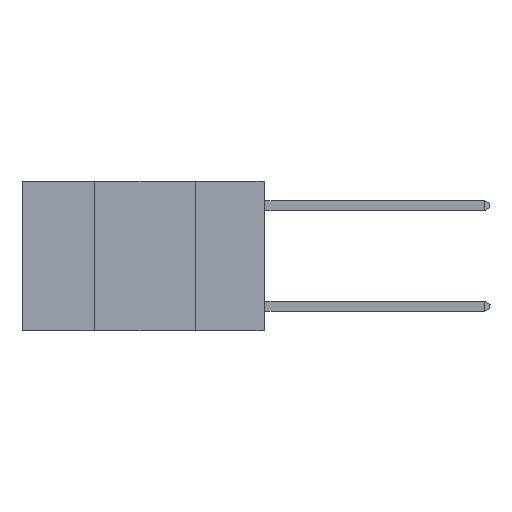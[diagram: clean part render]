
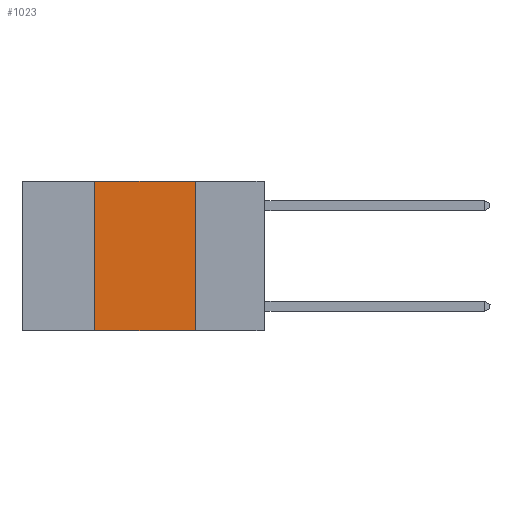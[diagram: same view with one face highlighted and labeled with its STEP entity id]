
A CAD part, left-side view. The second image highlights one B-rep face of the part: STEP entity #1023.
In plain terms, the highlighted planar face has unit normal (-1, 0, 0).
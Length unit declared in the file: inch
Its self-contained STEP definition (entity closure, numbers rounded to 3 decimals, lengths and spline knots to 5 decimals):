
#689 = VERTEX_POINT ( 'NONE', #1444 ) ;
#740 = PLANE ( 'NONE',  #11477 ) ;
#893 = ORIENTED_EDGE ( 'NONE', *, *, #12633, .T. ) ;
#1023 = ADVANCED_FACE ( 'NONE', ( #6993 ), #740, .F. ) ;
#1025 = LINE ( 'NONE', #11976, #3713 ) ;
#1444 = CARTESIAN_POINT ( 'NONE',  ( 0., 0.17, -0.37 ) ) ;
#2032 = VERTEX_POINT ( 'NONE', #9055 ) ;
#2495 = VERTEX_POINT ( 'NONE', #12577 ) ;
#2606 = DIRECTION ( 'NONE',  ( 0., 0., -1. ) ) ;
#3270 = DIRECTION ( 'NONE',  ( 0., -1., 0. ) ) ;
#3518 = DIRECTION ( 'NONE',  ( 1., 0., 0. ) ) ;
#3713 = VECTOR ( 'NONE', #3270, 39.37008 ) ;
#4757 = VECTOR ( 'NONE', #5237, 39.37008 ) ;
#5237 = DIRECTION ( 'NONE',  ( 0., 0., 1. ) ) ;
#6869 = DIRECTION ( 'NONE',  ( 0., 0., -1. ) ) ;
#6993 = FACE_OUTER_BOUND ( 'NONE', #9588, .T. ) ;
#7003 = CARTESIAN_POINT ( 'NONE',  ( 0., 0.17, 0. ) ) ;
#7303 = CARTESIAN_POINT ( 'NONE',  ( 0., 0.6, 0. ) ) ;
#7320 = EDGE_CURVE ( 'NONE', #9638, #2032, #7602, .T. ) ;
#7572 = LINE ( 'NONE', #8817, #12951 ) ;
#7602 = LINE ( 'NONE', #12679, #4757 ) ;
#7935 = CARTESIAN_POINT ( 'NONE',  ( 0., 0.42, -0.37 ) ) ;
#8469 = EDGE_CURVE ( 'NONE', #2032, #2495, #7572, .T. ) ;
#8770 = EDGE_CURVE ( 'NONE', #2495, #689, #9926, .T. ) ;
#8817 = CARTESIAN_POINT ( 'NONE',  ( 0., 0.6, 0. ) ) ;
#9055 = CARTESIAN_POINT ( 'NONE',  ( 0., 0.42, 0. ) ) ;
#9588 = EDGE_LOOP ( 'NONE', ( #13943, #11713, #11578, #893 ) ) ;
#9638 = VERTEX_POINT ( 'NONE', #7935 ) ;
#9894 = DIRECTION ( 'NONE',  ( 0., -1., 0. ) ) ;
#9926 = LINE ( 'NONE', #7003, #12454 ) ;
#11477 = AXIS2_PLACEMENT_3D ( 'NONE', #7303, #3518, #6869 ) ;
#11578 = ORIENTED_EDGE ( 'NONE', *, *, #7320, .F. ) ;
#11713 = ORIENTED_EDGE ( 'NONE', *, *, #8469, .F. ) ;
#11976 = CARTESIAN_POINT ( 'NONE',  ( 0., 0.6, -0.37 ) ) ;
#12454 = VECTOR ( 'NONE', #2606, 39.37008 ) ;
#12577 = CARTESIAN_POINT ( 'NONE',  ( 0., 0.17, 0. ) ) ;
#12633 = EDGE_CURVE ( 'NONE', #9638, #689, #1025, .T. ) ;
#12679 = CARTESIAN_POINT ( 'NONE',  ( 0., 0.42, 0. ) ) ;
#12951 = VECTOR ( 'NONE', #9894, 39.37008 ) ;
#13943 = ORIENTED_EDGE ( 'NONE', *, *, #8770, .F. ) ;
